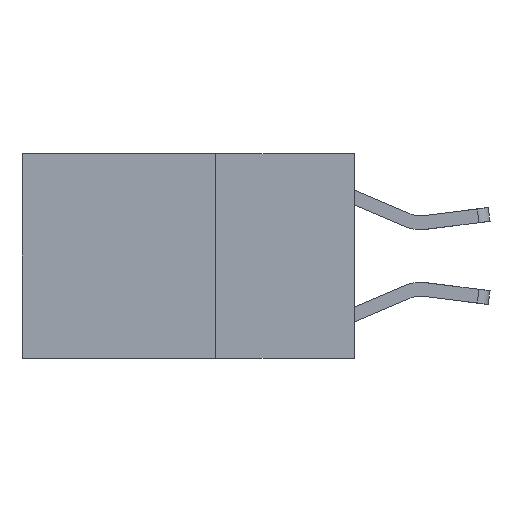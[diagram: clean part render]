
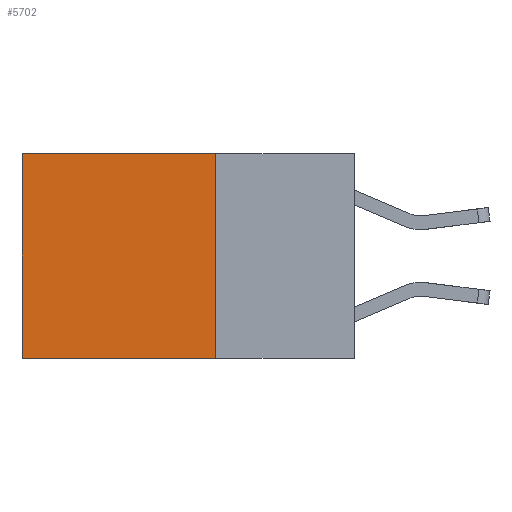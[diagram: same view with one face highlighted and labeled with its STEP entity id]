
A CAD part, left-side view. The second image highlights one B-rep face of the part: STEP entity #5702.
In plain terms, the highlighted planar face has unit normal (-1, 0, 0).
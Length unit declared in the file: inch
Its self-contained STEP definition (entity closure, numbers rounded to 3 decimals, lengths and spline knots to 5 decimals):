
#40 = VECTOR ( 'NONE', #7067, 39.37008 ) ;
#211 = EDGE_CURVE ( 'NONE', #1298, #3418, #1798, .T. ) ;
#371 = CARTESIAN_POINT ( 'NONE',  ( 0.2625, 0.25, 0. ) ) ;
#532 = VECTOR ( 'NONE', #2443, 39.37008 ) ;
#852 = CARTESIAN_POINT ( 'NONE',  ( 0.2625, 0.25, 0. ) ) ;
#1298 = VERTEX_POINT ( 'NONE', #3180 ) ;
#1677 = ORIENTED_EDGE ( 'NONE', *, *, #4909, .T. ) ;
#1737 = CARTESIAN_POINT ( 'NONE',  ( 0.2625, 0.25, 0. ) ) ;
#1798 = LINE ( 'NONE', #852, #40 ) ;
#2443 = DIRECTION ( 'NONE',  ( 0., 0., -1. ) ) ;
#3117 = ORIENTED_EDGE ( 'NONE', *, *, #4281, .F. ) ;
#3180 = CARTESIAN_POINT ( 'NONE',  ( 0.2625, 0.25, 0. ) ) ;
#3418 = VERTEX_POINT ( 'NONE', #4132 ) ;
#3591 = DIRECTION ( 'NONE',  ( 0., 1., 0. ) ) ;
#3747 = EDGE_LOOP ( 'NONE', ( #1677, #3117, #5172, #10155 ) ) ;
#3822 = PLANE ( 'NONE',  #6363 ) ;
#4132 = CARTESIAN_POINT ( 'NONE',  ( 0.2625, 0.6, 0. ) ) ;
#4254 = VERTEX_POINT ( 'NONE', #8015 ) ;
#4281 = EDGE_CURVE ( 'NONE', #4254, #5920, #5536, .T. ) ;
#4413 = LINE ( 'NONE', #1737, #7209 ) ;
#4743 = LINE ( 'NONE', #8347, #532 ) ;
#4909 = EDGE_CURVE ( 'NONE', #3418, #5920, #4743, .T. ) ;
#5172 = ORIENTED_EDGE ( 'NONE', *, *, #10494, .F. ) ;
#5536 = LINE ( 'NONE', #7116, #5584 ) ;
#5584 = VECTOR ( 'NONE', #3591, 39.37008 ) ;
#5702 = ADVANCED_FACE ( 'NONE', ( #10106 ), #3822, .F. ) ;
#5920 = VERTEX_POINT ( 'NONE', #9979 ) ;
#6312 = DIRECTION ( 'NONE',  ( 0., 0., -1. ) ) ;
#6363 = AXIS2_PLACEMENT_3D ( 'NONE', #371, #7399, #11008 ) ;
#7067 = DIRECTION ( 'NONE',  ( 0., 1., 0. ) ) ;
#7116 = CARTESIAN_POINT ( 'NONE',  ( 0.2625, 0.25, -0.37 ) ) ;
#7209 = VECTOR ( 'NONE', #6312, 39.37008 ) ;
#7399 = DIRECTION ( 'NONE',  ( 1., 0., 0. ) ) ;
#8015 = CARTESIAN_POINT ( 'NONE',  ( 0.2625, 0.25, -0.37 ) ) ;
#8347 = CARTESIAN_POINT ( 'NONE',  ( 0.2625, 0.6, 0. ) ) ;
#9979 = CARTESIAN_POINT ( 'NONE',  ( 0.2625, 0.6, -0.37 ) ) ;
#10106 = FACE_OUTER_BOUND ( 'NONE', #3747, .T. ) ;
#10155 = ORIENTED_EDGE ( 'NONE', *, *, #211, .T. ) ;
#10494 = EDGE_CURVE ( 'NONE', #1298, #4254, #4413, .T. ) ;
#11008 = DIRECTION ( 'NONE',  ( 0., 0., -1. ) ) ;
